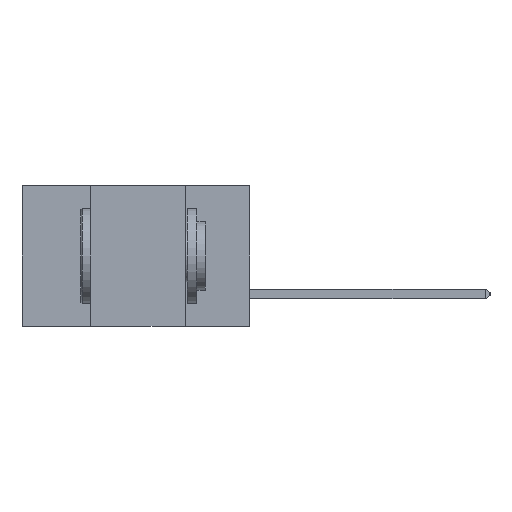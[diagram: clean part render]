
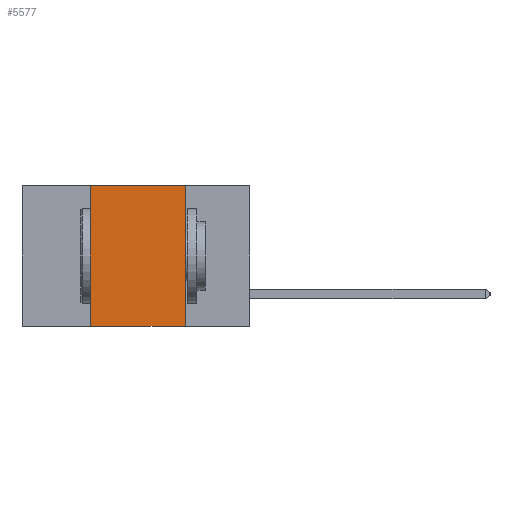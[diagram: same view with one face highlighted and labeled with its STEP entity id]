
A CAD part, left-side view. The second image highlights one B-rep face of the part: STEP entity #5577.
In plain terms, the highlighted planar face has unit normal (-1, 0, 0).
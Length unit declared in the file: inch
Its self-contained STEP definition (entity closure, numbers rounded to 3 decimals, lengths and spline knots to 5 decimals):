
#10 = CARTESIAN_POINT ( 'NONE',  ( 0., 0.6, 0. ) ) ;
#69 = FACE_OUTER_BOUND ( 'NONE', #8027, .T. ) ;
#88 = ORIENTED_EDGE ( 'NONE', *, *, #734, .F. ) ;
#215 = LINE ( 'NONE', #15916, #7111 ) ;
#542 = ORIENTED_EDGE ( 'NONE', *, *, #7671, .T. ) ;
#629 = DIRECTION ( 'NONE',  ( 0., -1., 0. ) ) ;
#653 = CARTESIAN_POINT ( 'NONE',  ( 0., 0.42, -0.37 ) ) ;
#734 = EDGE_CURVE ( 'NONE', #7391, #15179, #215, .T. ) ;
#993 = CARTESIAN_POINT ( 'NONE',  ( 0., 0.6, 0. ) ) ;
#1834 = VECTOR ( 'NONE', #8071, 39.37008 ) ;
#1874 = LINE ( 'NONE', #993, #5880 ) ;
#2291 = CARTESIAN_POINT ( 'NONE',  ( 0., 0.17, 0. ) ) ;
#2908 = EDGE_CURVE ( 'NONE', #15766, #7391, #1874, .T. ) ;
#3441 = DIRECTION ( 'NONE',  ( 0., 0., 1. ) ) ;
#3604 = CARTESIAN_POINT ( 'NONE',  ( 0., 0.42, 0. ) ) ;
#4327 = PLANE ( 'NONE',  #10580 ) ;
#4489 = EDGE_CURVE ( 'NONE', #13837, #15766, #7450, .T. ) ;
#5577 = ADVANCED_FACE ( 'NONE', ( #69 ), #4327, .F. ) ;
#5656 = DIRECTION ( 'NONE',  ( 0., 0., -1. ) ) ;
#5880 = VECTOR ( 'NONE', #629, 39.37008 ) ;
#7111 = VECTOR ( 'NONE', #11682, 39.37008 ) ;
#7391 = VERTEX_POINT ( 'NONE', #2291 ) ;
#7450 = LINE ( 'NONE', #3604, #13437 ) ;
#7671 = EDGE_CURVE ( 'NONE', #13837, #15179, #9179, .T. ) ;
#8027 = EDGE_LOOP ( 'NONE', ( #88, #11228, #12263, #542 ) ) ;
#8071 = DIRECTION ( 'NONE',  ( 0., -1., 0. ) ) ;
#8838 = CARTESIAN_POINT ( 'NONE',  ( 0., 0.42, 0. ) ) ;
#9179 = LINE ( 'NONE', #13979, #1834 ) ;
#10580 = AXIS2_PLACEMENT_3D ( 'NONE', #10, #12983, #5656 ) ;
#11228 = ORIENTED_EDGE ( 'NONE', *, *, #2908, .F. ) ;
#11619 = CARTESIAN_POINT ( 'NONE',  ( 0., 0.17, -0.37 ) ) ;
#11682 = DIRECTION ( 'NONE',  ( 0., 0., -1. ) ) ;
#12263 = ORIENTED_EDGE ( 'NONE', *, *, #4489, .F. ) ;
#12983 = DIRECTION ( 'NONE',  ( 1., 0., 0. ) ) ;
#13437 = VECTOR ( 'NONE', #3441, 39.37008 ) ;
#13837 = VERTEX_POINT ( 'NONE', #653 ) ;
#13979 = CARTESIAN_POINT ( 'NONE',  ( 0., 0.6, -0.37 ) ) ;
#15179 = VERTEX_POINT ( 'NONE', #11619 ) ;
#15766 = VERTEX_POINT ( 'NONE', #8838 ) ;
#15916 = CARTESIAN_POINT ( 'NONE',  ( 0., 0.17, 0. ) ) ;
